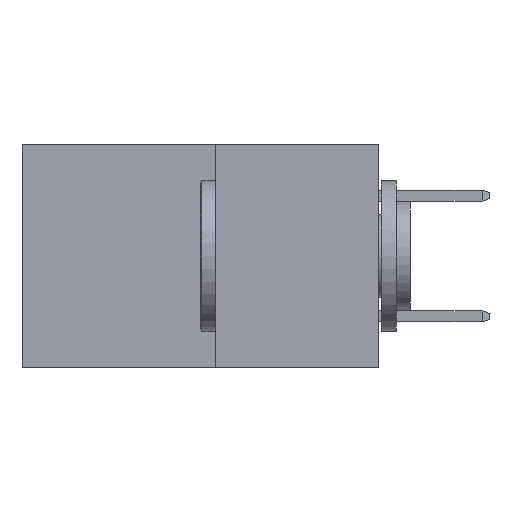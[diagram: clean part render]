
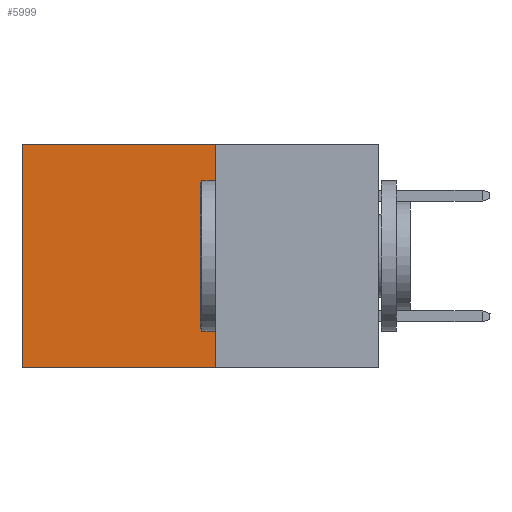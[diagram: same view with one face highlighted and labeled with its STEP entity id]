
A CAD part, left-side view. The second image highlights one B-rep face of the part: STEP entity #5999.
In plain terms, the highlighted planar face has unit normal (-1, 0, 0).
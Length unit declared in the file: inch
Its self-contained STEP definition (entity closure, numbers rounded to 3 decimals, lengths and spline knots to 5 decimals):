
#462 = CARTESIAN_POINT ( 'NONE',  ( 0.277, 0.27, -0.37 ) ) ;
#695 = EDGE_CURVE ( 'NONE', #5000, #7175, #2324, .T. ) ;
#742 = EDGE_CURVE ( 'NONE', #6259, #902, #1528, .T. ) ;
#868 = DIRECTION ( 'NONE',  ( 0., 0., -1. ) ) ;
#902 = VERTEX_POINT ( 'NONE', #8598 ) ;
#1029 = EDGE_CURVE ( 'NONE', #5000, #6259, #6147, .T. ) ;
#1528 = LINE ( 'NONE', #6975, #4855 ) ;
#2161 = EDGE_CURVE ( 'NONE', #7175, #902, #5478, .T. ) ;
#2324 = LINE ( 'NONE', #5253, #5612 ) ;
#2468 = EDGE_LOOP ( 'NONE', ( #4875, #7834, #8299, #7328 ) ) ;
#2515 = VECTOR ( 'NONE', #8043, 39.37008 ) ;
#2516 = CARTESIAN_POINT ( 'NONE',  ( 0.277, 0.59, 0. ) ) ;
#2622 = CARTESIAN_POINT ( 'NONE',  ( 0.277, 0.27, -0.37 ) ) ;
#2706 = FACE_OUTER_BOUND ( 'NONE', #2468, .T. ) ;
#3339 = DIRECTION ( 'NONE',  ( 0., 1., 0. ) ) ;
#3844 = PLANE ( 'NONE',  #7848 ) ;
#3981 = DIRECTION ( 'NONE',  ( 0., 1., 0. ) ) ;
#4752 = CARTESIAN_POINT ( 'NONE',  ( 0.277, 0.27, 0. ) ) ;
#4855 = VECTOR ( 'NONE', #3339, 39.37008 ) ;
#4875 = ORIENTED_EDGE ( 'NONE', *, *, #2161, .T. ) ;
#5000 = VERTEX_POINT ( 'NONE', #4752 ) ;
#5167 = DIRECTION ( 'NONE',  ( 1., 0., 0. ) ) ;
#5253 = CARTESIAN_POINT ( 'NONE',  ( 0.277, 0.27, 0. ) ) ;
#5478 = LINE ( 'NONE', #6767, #6671 ) ;
#5612 = VECTOR ( 'NONE', #3981, 39.37008 ) ;
#5999 = ADVANCED_FACE ( 'NONE', ( #2706 ), #3844, .F. ) ;
#6147 = LINE ( 'NONE', #462, #2515 ) ;
#6259 = VERTEX_POINT ( 'NONE', #2622 ) ;
#6671 = VECTOR ( 'NONE', #6806, 39.37008 ) ;
#6767 = CARTESIAN_POINT ( 'NONE',  ( 0.277, 0.59, -0.37 ) ) ;
#6806 = DIRECTION ( 'NONE',  ( 0., 0., -1. ) ) ;
#6912 = CARTESIAN_POINT ( 'NONE',  ( 0.277, 0.27, -0.37 ) ) ;
#6975 = CARTESIAN_POINT ( 'NONE',  ( 0.277, 0.27, -0.37 ) ) ;
#7175 = VERTEX_POINT ( 'NONE', #2516 ) ;
#7328 = ORIENTED_EDGE ( 'NONE', *, *, #695, .T. ) ;
#7834 = ORIENTED_EDGE ( 'NONE', *, *, #742, .F. ) ;
#7848 = AXIS2_PLACEMENT_3D ( 'NONE', #6912, #5167, #868 ) ;
#8043 = DIRECTION ( 'NONE',  ( 0., 0., -1. ) ) ;
#8299 = ORIENTED_EDGE ( 'NONE', *, *, #1029, .F. ) ;
#8598 = CARTESIAN_POINT ( 'NONE',  ( 0.277, 0.59, -0.37 ) ) ;
